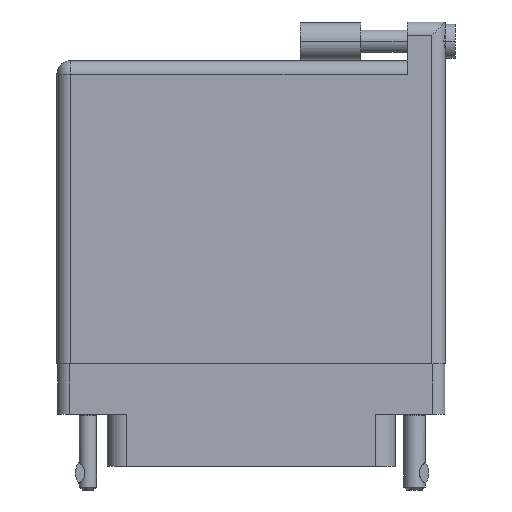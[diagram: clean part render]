
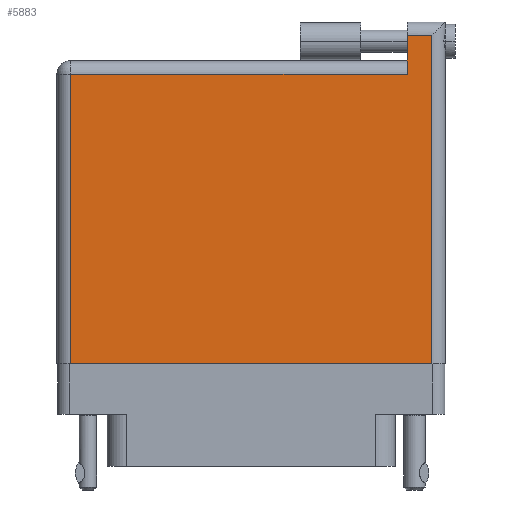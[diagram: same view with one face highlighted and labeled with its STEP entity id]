
A CAD part, front view. The second image highlights one B-rep face of the part: STEP entity #5883.
In plain terms, the highlighted face is planar.
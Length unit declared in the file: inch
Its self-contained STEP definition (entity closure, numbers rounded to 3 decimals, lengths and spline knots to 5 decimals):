
#1075 = CARTESIAN_POINT ( 'NONE',  ( 1.811, 1.696, 0. ) ) ;
#1461 = EDGE_LOOP ( 'NONE', ( #4730, #28540, #23453, #39552, #19183, #31876 ) ) ;
#2311 = LINE ( 'NONE', #34054, #43496 ) ;
#2597 = EDGE_CURVE ( 'NONE', #17777, #2638, #18816, .T. ) ;
#2638 = VERTEX_POINT ( 'NONE', #11090 ) ;
#3571 = EDGE_CURVE ( 'NONE', #15668, #32994, #29752, .T. ) ;
#4730 = ORIENTED_EDGE ( 'NONE', *, *, #31711, .T. ) ;
#5883 = ADVANCED_FACE ( 'NONE', ( #12916 ), #16956, .F. ) ;
#8611 = AXIS2_PLACEMENT_3D ( 'NONE', #46190, #27651, #38809 ) ;
#8679 = DIRECTION ( 'NONE',  ( 0., -1., 0. ) ) ;
#8937 = DIRECTION ( 'NONE',  ( 0., 1., 0. ) ) ;
#10057 = VECTOR ( 'NONE', #8679, 39.37008 ) ;
#11090 = CARTESIAN_POINT ( 'NONE',  ( 0.07, 0., 0. ) ) ;
#12916 = FACE_OUTER_BOUND ( 'NONE', #1461, .T. ) ;
#14373 = EDGE_CURVE ( 'NONE', #22660, #15668, #22000, .T. ) ;
#14756 = VECTOR ( 'NONE', #19523, 39.37008 ) ;
#15668 = VERTEX_POINT ( 'NONE', #1075 ) ;
#16956 = PLANE ( 'NONE',  #8611 ) ;
#17028 = VECTOR ( 'NONE', #40468, 39.37008 ) ;
#17777 = VERTEX_POINT ( 'NONE', #28582 ) ;
#18172 = LINE ( 'NONE', #44008, #17028 ) ;
#18187 = VECTOR ( 'NONE', #47502, 39.37008 ) ;
#18816 = LINE ( 'NONE', #26356, #14756 ) ;
#19183 = ORIENTED_EDGE ( 'NONE', *, *, #42544, .T. ) ;
#19523 = DIRECTION ( 'NONE',  ( 0., -1., 0. ) ) ;
#20822 = VECTOR ( 'NONE', #43499, 39.37008 ) ;
#21098 = CARTESIAN_POINT ( 'NONE',  ( 1.938, 0., 0. ) ) ;
#22000 = LINE ( 'NONE', #40129, #20822 ) ;
#22660 = VERTEX_POINT ( 'NONE', #28724 ) ;
#23453 = ORIENTED_EDGE ( 'NONE', *, *, #14373, .T. ) ;
#26356 = CARTESIAN_POINT ( 'NONE',  ( 0.07, 0., 0. ) ) ;
#26966 = VERTEX_POINT ( 'NONE', #21098 ) ;
#27651 = DIRECTION ( 'NONE',  ( 0., 0., -1. ) ) ;
#28540 = ORIENTED_EDGE ( 'NONE', *, *, #36667, .T. ) ;
#28582 = CARTESIAN_POINT ( 'NONE',  ( 0.07, 1.496, 0. ) ) ;
#28724 = CARTESIAN_POINT ( 'NONE',  ( 1.938, 1.696, 0. ) ) ;
#29752 = LINE ( 'NONE', #38163, #10057 ) ;
#31711 = EDGE_CURVE ( 'NONE', #2638, #26966, #43657, .T. ) ;
#31876 = ORIENTED_EDGE ( 'NONE', *, *, #2597, .T. ) ;
#32994 = VERTEX_POINT ( 'NONE', #44593 ) ;
#34054 = CARTESIAN_POINT ( 'NONE',  ( 1.938, 1.766, 0. ) ) ;
#36667 = EDGE_CURVE ( 'NONE', #26966, #22660, #2311, .T. ) ;
#38163 = CARTESIAN_POINT ( 'NONE',  ( 1.811, 1.766, 0. ) ) ;
#38809 = DIRECTION ( 'NONE',  ( -1., 0., 0. ) ) ;
#39552 = ORIENTED_EDGE ( 'NONE', *, *, #3571, .T. ) ;
#40129 = CARTESIAN_POINT ( 'NONE',  ( 0., 1.696, 0. ) ) ;
#40468 = DIRECTION ( 'NONE',  ( -1., 0., 0. ) ) ;
#42544 = EDGE_CURVE ( 'NONE', #32994, #17777, #18172, .T. ) ;
#43152 = CARTESIAN_POINT ( 'NONE',  ( 0., 0., 0. ) ) ;
#43496 = VECTOR ( 'NONE', #8937, 39.37008 ) ;
#43499 = DIRECTION ( 'NONE',  ( -1., 0., 0. ) ) ;
#43657 = LINE ( 'NONE', #43152, #18187 ) ;
#44008 = CARTESIAN_POINT ( 'NONE',  ( 0., 1.496, 0. ) ) ;
#44593 = CARTESIAN_POINT ( 'NONE',  ( 1.811, 1.496, 0. ) ) ;
#46190 = CARTESIAN_POINT ( 'NONE',  ( 0., 1.566, 0. ) ) ;
#47502 = DIRECTION ( 'NONE',  ( 1., 0., 0. ) ) ;
